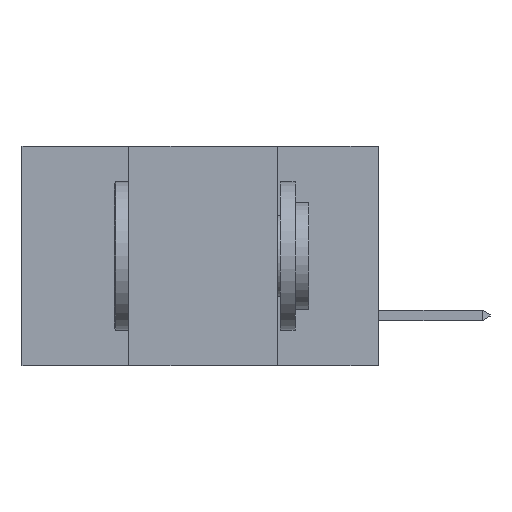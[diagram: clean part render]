
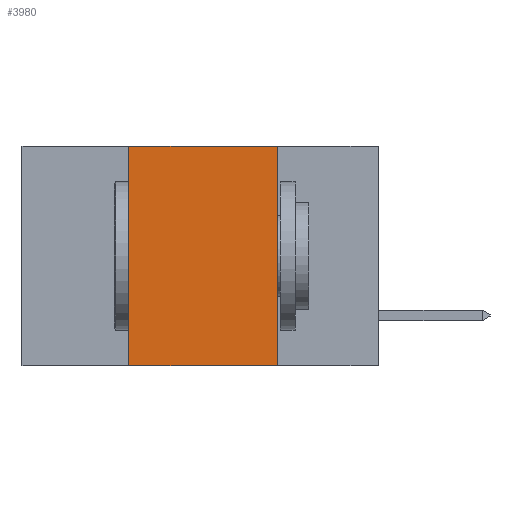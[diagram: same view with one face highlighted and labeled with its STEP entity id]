
A CAD part, left-side view. The second image highlights one B-rep face of the part: STEP entity #3980.
In plain terms, the highlighted planar face has unit normal (-1, 0, 0).
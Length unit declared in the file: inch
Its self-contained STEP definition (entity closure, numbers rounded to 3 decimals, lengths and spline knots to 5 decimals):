
#362 = VECTOR ( 'NONE', #5016, 39.37008 ) ;
#637 = ORIENTED_EDGE ( 'NONE', *, *, #1696, .F. ) ;
#1247 = CARTESIAN_POINT ( 'NONE',  ( 0., 0.17, -0.37 ) ) ;
#1696 = EDGE_CURVE ( 'NONE', #7814, #7014, #3564, .T. ) ;
#1791 = LINE ( 'NONE', #8505, #9561 ) ;
#1918 = CARTESIAN_POINT ( 'NONE',  ( 0., 0.6, 0. ) ) ;
#2103 = DIRECTION ( 'NONE',  ( 0., 0., -1. ) ) ;
#2277 = DIRECTION ( 'NONE',  ( 0., -1., 0. ) ) ;
#2309 = DIRECTION ( 'NONE',  ( 1., 0., 0. ) ) ;
#2465 = FACE_OUTER_BOUND ( 'NONE', #4021, .T. ) ;
#2576 = LINE ( 'NONE', #4254, #362 ) ;
#2685 = PLANE ( 'NONE',  #9901 ) ;
#2737 = CARTESIAN_POINT ( 'NONE',  ( 0., 0.6, 0. ) ) ;
#3417 = ORIENTED_EDGE ( 'NONE', *, *, #9636, .F. ) ;
#3564 = LINE ( 'NONE', #7805, #7222 ) ;
#3980 = ADVANCED_FACE ( 'NONE', ( #2465 ), #2685, .F. ) ;
#4021 = EDGE_LOOP ( 'NONE', ( #637, #6703, #3417, #5192 ) ) ;
#4220 = LINE ( 'NONE', #1918, #8103 ) ;
#4254 = CARTESIAN_POINT ( 'NONE',  ( 0., 0.42, -0.37 ) ) ;
#4290 = DIRECTION ( 'NONE',  ( 0., -1., 0. ) ) ;
#5016 = DIRECTION ( 'NONE',  ( 0., 0., 1. ) ) ;
#5192 = ORIENTED_EDGE ( 'NONE', *, *, #6471, .T. ) ;
#6471 = EDGE_CURVE ( 'NONE', #8790, #7014, #1791, .T. ) ;
#6703 = ORIENTED_EDGE ( 'NONE', *, *, #9684, .F. ) ;
#7014 = VERTEX_POINT ( 'NONE', #1247 ) ;
#7222 = VECTOR ( 'NONE', #8324, 39.37008 ) ;
#7674 = CARTESIAN_POINT ( 'NONE',  ( 0., 0.42, -0.37 ) ) ;
#7805 = CARTESIAN_POINT ( 'NONE',  ( 0., 0.17, -0.37 ) ) ;
#7814 = VERTEX_POINT ( 'NONE', #9514 ) ;
#7904 = VERTEX_POINT ( 'NONE', #9607 ) ;
#8103 = VECTOR ( 'NONE', #4290, 39.37008 ) ;
#8324 = DIRECTION ( 'NONE',  ( 0., 0., -1. ) ) ;
#8505 = CARTESIAN_POINT ( 'NONE',  ( 0., 0.6, -0.37 ) ) ;
#8790 = VERTEX_POINT ( 'NONE', #7674 ) ;
#9514 = CARTESIAN_POINT ( 'NONE',  ( 0., 0.17, 0. ) ) ;
#9561 = VECTOR ( 'NONE', #2277, 39.37008 ) ;
#9607 = CARTESIAN_POINT ( 'NONE',  ( 0., 0.42, 0. ) ) ;
#9636 = EDGE_CURVE ( 'NONE', #8790, #7904, #2576, .T. ) ;
#9684 = EDGE_CURVE ( 'NONE', #7904, #7814, #4220, .T. ) ;
#9901 = AXIS2_PLACEMENT_3D ( 'NONE', #2737, #2309, #2103 ) ;
